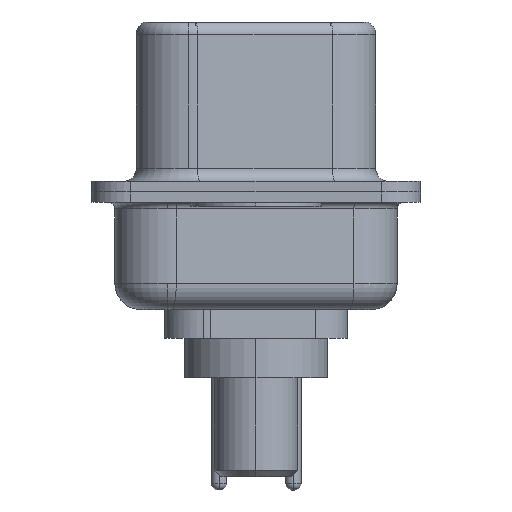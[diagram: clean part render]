
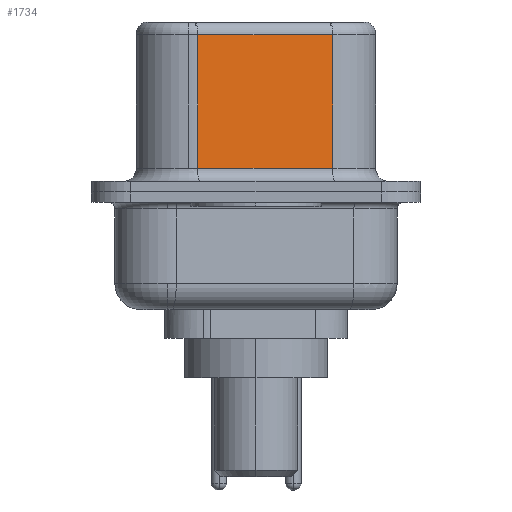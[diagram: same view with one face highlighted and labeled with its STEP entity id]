
A CAD part, left-side view. The second image highlights one B-rep face of the part: STEP entity #1734.
In plain terms, the highlighted planar face has unit normal (-0.985, -0.174, 0).
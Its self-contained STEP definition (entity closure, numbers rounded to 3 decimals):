
#208 = PLANE ( 'NONE',  #1492 ) ;
#1409 = VECTOR ( 'NONE', #13835, 1000. ) ;
#1492 = AXIS2_PLACEMENT_3D ( 'NONE', #16651, #6838, #3950 ) ;
#1734 = ADVANCED_FACE ( 'NONE', ( #17914 ), #208, .F. ) ;
#2722 = CARTESIAN_POINT ( 'NONE',  ( 4.58, -2.927, 0.9 ) ) ;
#3358 = LINE ( 'NONE', #10195, #11087 ) ;
#3603 = ORIENTED_EDGE ( 'NONE', *, *, #4951, .F. ) ;
#3913 = DIRECTION ( 'NONE',  ( -0.174, 0.985, 0. ) ) ;
#3950 = DIRECTION ( 'NONE',  ( -0.174, 0.985, 0. ) ) ;
#4155 = CARTESIAN_POINT ( 'NONE',  ( 4.58, -2.927, 6.02 ) ) ;
#4857 = VERTEX_POINT ( 'NONE', #17056 ) ;
#4951 = EDGE_CURVE ( 'NONE', #19182, #4857, #3358, .T. ) ;
#6140 = VECTOR ( 'NONE', #3913, 1000. ) ;
#6258 = EDGE_CURVE ( 'NONE', #19182, #8836, #17774, .T. ) ;
#6386 = LINE ( 'NONE', #2722, #10571 ) ;
#6838 = DIRECTION ( 'NONE',  ( 0.985, 0.174, 0. ) ) ;
#7253 = VERTEX_POINT ( 'NONE', #15523 ) ;
#8306 = EDGE_CURVE ( 'NONE', #7253, #4857, #6386, .T. ) ;
#8836 = VERTEX_POINT ( 'NONE', #18664 ) ;
#10195 = CARTESIAN_POINT ( 'NONE',  ( 4.58, -2.927, 6.52 ) ) ;
#10571 = VECTOR ( 'NONE', #10632, 1000. ) ;
#10632 = DIRECTION ( 'NONE',  ( 0.174, -0.985, 0. ) ) ;
#10695 = ORIENTED_EDGE ( 'NONE', *, *, #15886, .T. ) ;
#10773 = CARTESIAN_POINT ( 'NONE',  ( 4.58, -2.927, 6.02 ) ) ;
#11087 = VECTOR ( 'NONE', #11521, 1000. ) ;
#11521 = DIRECTION ( 'NONE',  ( 0., 0., -1. ) ) ;
#12083 = ORIENTED_EDGE ( 'NONE', *, *, #8306, .T. ) ;
#12760 = EDGE_LOOP ( 'NONE', ( #3603, #12909, #10695, #12083 ) ) ;
#12909 = ORIENTED_EDGE ( 'NONE', *, *, #6258, .T. ) ;
#13835 = DIRECTION ( 'NONE',  ( 0., 0., -1. ) ) ;
#15523 = CARTESIAN_POINT ( 'NONE',  ( 3.67, 2.233, 0.9 ) ) ;
#15886 = EDGE_CURVE ( 'NONE', #8836, #7253, #17127, .T. ) ;
#16651 = CARTESIAN_POINT ( 'NONE',  ( 4.58, -2.927, 6.52 ) ) ;
#17056 = CARTESIAN_POINT ( 'NONE',  ( 4.58, -2.927, 0.9 ) ) ;
#17127 = LINE ( 'NONE', #18181, #1409 ) ;
#17774 = LINE ( 'NONE', #10773, #6140 ) ;
#17914 = FACE_OUTER_BOUND ( 'NONE', #12760, .T. ) ;
#18181 = CARTESIAN_POINT ( 'NONE',  ( 3.67, 2.233, 6.52 ) ) ;
#18664 = CARTESIAN_POINT ( 'NONE',  ( 3.67, 2.233, 6.02 ) ) ;
#19182 = VERTEX_POINT ( 'NONE', #4155 ) ;
